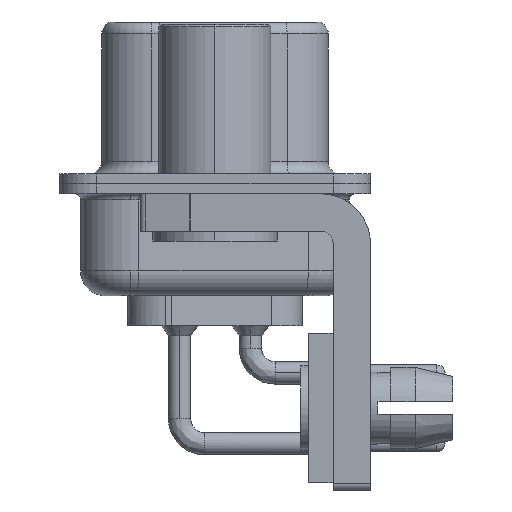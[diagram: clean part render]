
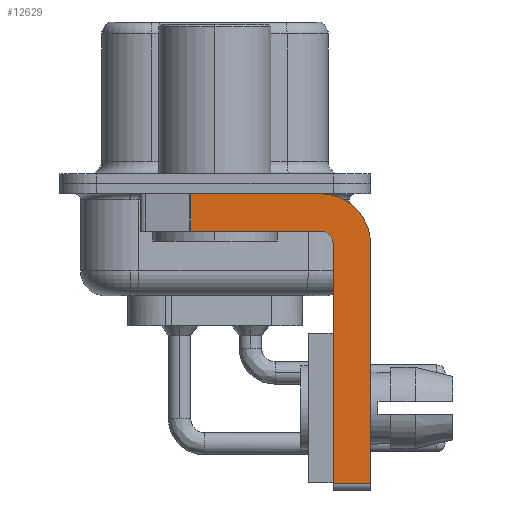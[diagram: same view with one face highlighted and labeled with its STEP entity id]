
A CAD part, left-side view. The second image highlights one B-rep face of the part: STEP entity #12629.
In plain terms, the highlighted planar face has unit normal (-1, 0, 0).
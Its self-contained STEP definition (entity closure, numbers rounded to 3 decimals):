
#12 = EDGE_CURVE ( 'NONE', #7099, #3313, #9861, .T. ) ;
#423 = DIRECTION ( 'NONE',  ( 0., 0., 1. ) ) ;
#667 = EDGE_CURVE ( 'NONE', #4431, #3313, #2062, .T. ) ;
#1837 = ORIENTED_EDGE ( 'NONE', *, *, #14012, .F. ) ;
#2062 = LINE ( 'NONE', #26672, #18222 ) ;
#2570 = VECTOR ( 'NONE', #13763, 1000. ) ;
#3313 = VERTEX_POINT ( 'NONE', #12931 ) ;
#4431 = VERTEX_POINT ( 'NONE', #8579 ) ;
#4449 = CIRCLE ( 'NONE', #25441, 2. ) ;
#4708 = ORIENTED_EDGE ( 'NONE', *, *, #4865, .F. ) ;
#4865 = EDGE_CURVE ( 'NONE', #11642, #26732, #8346, .T. ) ;
#5199 = CIRCLE ( 'NONE', #10427, 0.5 ) ;
#6425 = VECTOR ( 'NONE', #16255, 1000. ) ;
#6852 = ORIENTED_EDGE ( 'NONE', *, *, #667, .F. ) ;
#7099 = VERTEX_POINT ( 'NONE', #7586 ) ;
#7303 = VERTEX_POINT ( 'NONE', #15554 ) ;
#7586 = CARTESIAN_POINT ( 'NONE',  ( -2.9, 0.978, -0.4 ) ) ;
#8346 = LINE ( 'NONE', #13899, #2570 ) ;
#8402 = LINE ( 'NONE', #11781, #24888 ) ;
#8579 = CARTESIAN_POINT ( 'NONE',  ( -2.9, -4.25, -1.9 ) ) ;
#9176 = VECTOR ( 'NONE', #13870, 1000. ) ;
#9659 = CARTESIAN_POINT ( 'NONE',  ( -2.9, -4.25, -2.4 ) ) ;
#9861 = LINE ( 'NONE', #12202, #9176 ) ;
#10157 = CARTESIAN_POINT ( 'NONE',  ( -2.9, -6.25, -2.4 ) ) ;
#10172 = CARTESIAN_POINT ( 'NONE',  ( -2.9, -4.25, -2.4 ) ) ;
#10254 = ORIENTED_EDGE ( 'NONE', *, *, #19674, .F. ) ;
#10309 = EDGE_CURVE ( 'NONE', #11642, #20714, #12140, .T. ) ;
#10427 = AXIS2_PLACEMENT_3D ( 'NONE', #25516, #13267, #423 ) ;
#10442 = CARTESIAN_POINT ( 'NONE',  ( -2.9, -4.75, -12.05 ) ) ;
#11642 = VERTEX_POINT ( 'NONE', #10442 ) ;
#11714 = PLANE ( 'NONE',  #15480 ) ;
#11781 = CARTESIAN_POINT ( 'NONE',  ( -2.9, 3., -0.4 ) ) ;
#12112 = ORIENTED_EDGE ( 'NONE', *, *, #12, .T. ) ;
#12140 = LINE ( 'NONE', #14238, #6425 ) ;
#12154 = VECTOR ( 'NONE', #22535, 1000. ) ;
#12202 = CARTESIAN_POINT ( 'NONE',  ( -2.9, 0.978, -1.9 ) ) ;
#12294 = DIRECTION ( 'NONE',  ( 0., 0., -1. ) ) ;
#12629 = ADVANCED_FACE ( 'NONE', ( #26656 ), #11714, .F. ) ;
#12810 = LINE ( 'NONE', #10157, #12154 ) ;
#12931 = CARTESIAN_POINT ( 'NONE',  ( -2.9, 0.978, -1.9 ) ) ;
#13254 = CARTESIAN_POINT ( 'NONE',  ( -2.9, -4.75, -2.4 ) ) ;
#13265 = ORIENTED_EDGE ( 'NONE', *, *, #20655, .F. ) ;
#13267 = DIRECTION ( 'NONE',  ( -1., 0., 0. ) ) ;
#13763 = DIRECTION ( 'NONE',  ( 0., 0., 1. ) ) ;
#13870 = DIRECTION ( 'NONE',  ( 0., 0., -1. ) ) ;
#13899 = CARTESIAN_POINT ( 'NONE',  ( -2.9, -4.75, -12.3 ) ) ;
#13914 = DIRECTION ( 'NONE',  ( 0., -1., 0. ) ) ;
#13935 = DIRECTION ( 'NONE',  ( 0., 0., -1. ) ) ;
#14012 = EDGE_CURVE ( 'NONE', #7099, #24068, #8402, .T. ) ;
#14238 = CARTESIAN_POINT ( 'NONE',  ( -2.9, -4.25, -12.05 ) ) ;
#15480 = AXIS2_PLACEMENT_3D ( 'NONE', #9659, #26199, #13935 ) ;
#15554 = CARTESIAN_POINT ( 'NONE',  ( -2.9, -6.25, -2.4 ) ) ;
#16255 = DIRECTION ( 'NONE',  ( 0., -1., 0. ) ) ;
#16779 = EDGE_LOOP ( 'NONE', ( #1837, #12112, #6852, #10254, #4708, #19382, #20839, #13265 ) ) ;
#18222 = VECTOR ( 'NONE', #26584, 1000. ) ;
#18557 = CARTESIAN_POINT ( 'NONE',  ( -2.9, -6.25, -12.05 ) ) ;
#19382 = ORIENTED_EDGE ( 'NONE', *, *, #10309, .T. ) ;
#19674 = EDGE_CURVE ( 'NONE', #26732, #4431, #5199, .T. ) ;
#20449 = CARTESIAN_POINT ( 'NONE',  ( -2.9, -4.25, -0.4 ) ) ;
#20655 = EDGE_CURVE ( 'NONE', #24068, #7303, #4449, .T. ) ;
#20714 = VERTEX_POINT ( 'NONE', #18557 ) ;
#20839 = ORIENTED_EDGE ( 'NONE', *, *, #22800, .F. ) ;
#22535 = DIRECTION ( 'NONE',  ( 0., 0., -1. ) ) ;
#22800 = EDGE_CURVE ( 'NONE', #7303, #20714, #12810, .T. ) ;
#24068 = VERTEX_POINT ( 'NONE', #20449 ) ;
#24566 = DIRECTION ( 'NONE',  ( 1., 0., 0. ) ) ;
#24888 = VECTOR ( 'NONE', #13914, 1000. ) ;
#25441 = AXIS2_PLACEMENT_3D ( 'NONE', #10172, #24566, #12294 ) ;
#25516 = CARTESIAN_POINT ( 'NONE',  ( -2.9, -4.25, -2.4 ) ) ;
#26199 = DIRECTION ( 'NONE',  ( 1., 0., 0. ) ) ;
#26584 = DIRECTION ( 'NONE',  ( 0., 1., 0. ) ) ;
#26656 = FACE_OUTER_BOUND ( 'NONE', #16779, .T. ) ;
#26672 = CARTESIAN_POINT ( 'NONE',  ( -2.9, -4.25, -1.9 ) ) ;
#26732 = VERTEX_POINT ( 'NONE', #13254 ) ;
